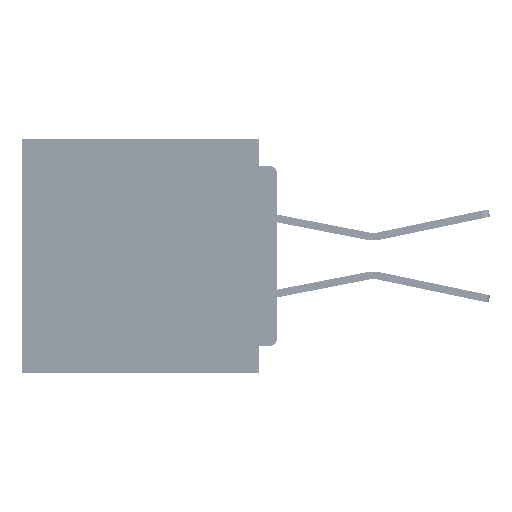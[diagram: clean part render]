
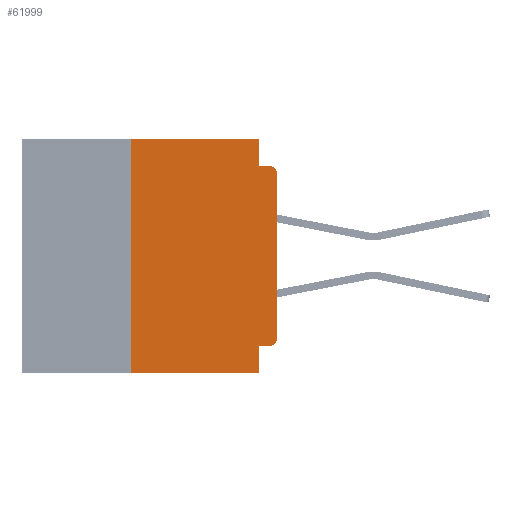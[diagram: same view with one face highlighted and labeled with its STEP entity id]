
A CAD part, left-side view. The second image highlights one B-rep face of the part: STEP entity #61999.
In plain terms, the highlighted planar face has unit normal (-1, 0, 0).
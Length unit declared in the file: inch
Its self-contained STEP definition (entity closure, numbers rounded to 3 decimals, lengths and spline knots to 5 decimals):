
#136 = CARTESIAN_POINT ( 'NONE',  ( 0., 0.25, 0. ) ) ;
#702 = DIRECTION ( 'NONE',  ( 0., 0., 1. ) ) ;
#851 = DIRECTION ( 'NONE',  ( -1., 0., 0. ) ) ;
#1193 = EDGE_CURVE ( 'NONE', #56111, #19656, #16438, .T. ) ;
#1339 = ORIENTED_EDGE ( 'NONE', *, *, #23417, .T. ) ;
#1462 = VECTOR ( 'NONE', #38180, 39.37008 ) ;
#2304 = VERTEX_POINT ( 'NONE', #56206 ) ;
#3399 = VECTOR ( 'NONE', #702, 39.37008 ) ;
#4113 = VECTOR ( 'NONE', #35135, 39.37008 ) ;
#4459 = DIRECTION ( 'NONE',  ( 1., 0., 0. ) ) ;
#5247 = ORIENTED_EDGE ( 'NONE', *, *, #41955, .F. ) ;
#6307 = EDGE_CURVE ( 'NONE', #49589, #40310, #62757, .T. ) ;
#6963 = ORIENTED_EDGE ( 'NONE', *, *, #1193, .F. ) ;
#8898 = CARTESIAN_POINT ( 'NONE',  ( 0., 0., -0.045 ) ) ;
#11327 = VERTEX_POINT ( 'NONE', #18063 ) ;
#13127 = ORIENTED_EDGE ( 'NONE', *, *, #51377, .F. ) ;
#13750 = LINE ( 'NONE', #61336, #63961 ) ;
#14013 = CIRCLE ( 'NONE', #24514, 0.015 ) ;
#14481 = ORIENTED_EDGE ( 'NONE', *, *, #58728, .F. ) ;
#15562 = VERTEX_POINT ( 'NONE', #31339 ) ;
#16078 = DIRECTION ( 'NONE',  ( -1., 0., 0. ) ) ;
#16438 = LINE ( 'NONE', #43015, #1462 ) ;
#18063 = CARTESIAN_POINT ( 'NONE',  ( 0., 0., -0.06 ) ) ;
#18684 = CARTESIAN_POINT ( 'NONE',  ( 0., 0.015, -0.045 ) ) ;
#18999 = ORIENTED_EDGE ( 'NONE', *, *, #6307, .T. ) ;
#19447 = LINE ( 'NONE', #32800, #29678 ) ;
#19462 = CARTESIAN_POINT ( 'NONE',  ( 0., 0.437, 0. ) ) ;
#19552 = CARTESIAN_POINT ( 'NONE',  ( 0., 0.031, 0. ) ) ;
#19656 = VERTEX_POINT ( 'NONE', #22319 ) ;
#21448 = FACE_OUTER_BOUND ( 'NONE', #26202, .T. ) ;
#21689 = CARTESIAN_POINT ( 'NONE',  ( 0., 0.25, -0.4 ) ) ;
#22319 = CARTESIAN_POINT ( 'NONE',  ( 0., 0.031, 0. ) ) ;
#22902 = DIRECTION ( 'NONE',  ( 0., 1., 0. ) ) ;
#23199 = CIRCLE ( 'NONE', #56171, 0.015 ) ;
#23417 = EDGE_CURVE ( 'NONE', #33600, #2304, #14013, .T. ) ;
#24514 = AXIS2_PLACEMENT_3D ( 'NONE', #46212, #16078, #51242 ) ;
#25986 = VECTOR ( 'NONE', #44781, 39.37008 ) ;
#26111 = EDGE_CURVE ( 'NONE', #2304, #11327, #31807, .T. ) ;
#26202 = EDGE_LOOP ( 'NONE', ( #62507, #61592, #13127, #57307, #6963, #5247, #18999, #32442, #14481, #1339 ) ) ;
#27563 = LINE ( 'NONE', #19552, #25986 ) ;
#29678 = VECTOR ( 'NONE', #22902, 39.37008 ) ;
#30860 = CARTESIAN_POINT ( 'NONE',  ( 0., 0.031, -0.4 ) ) ;
#31057 = CARTESIAN_POINT ( 'NONE',  ( 0., 0.015, -0.06 ) ) ;
#31339 = CARTESIAN_POINT ( 'NONE',  ( 0., 0.031, -0.355 ) ) ;
#31807 = LINE ( 'NONE', #50859, #3399 ) ;
#32442 = ORIENTED_EDGE ( 'NONE', *, *, #59871, .F. ) ;
#32800 = CARTESIAN_POINT ( 'NONE',  ( 0., 0., -0.355 ) ) ;
#33600 = VERTEX_POINT ( 'NONE', #63336 ) ;
#34626 = PLANE ( 'NONE',  #52569 ) ;
#34887 = DIRECTION ( 'NONE',  ( 0., -1., 0. ) ) ;
#35135 = DIRECTION ( 'NONE',  ( 0., 0., 1. ) ) ;
#36077 = DIRECTION ( 'NONE',  ( 0., 0., -1. ) ) ;
#36123 = VECTOR ( 'NONE', #34887, 39.37008 ) ;
#38180 = DIRECTION ( 'NONE',  ( 0., -1., 0. ) ) ;
#39653 = DIRECTION ( 'NONE',  ( 0., 0., -1. ) ) ;
#39913 = CARTESIAN_POINT ( 'NONE',  ( 0., 0.437, -0.4 ) ) ;
#40310 = VERTEX_POINT ( 'NONE', #30860 ) ;
#41955 = EDGE_CURVE ( 'NONE', #49589, #56111, #42657, .T. ) ;
#42657 = LINE ( 'NONE', #65091, #4113 ) ;
#43015 = CARTESIAN_POINT ( 'NONE',  ( 0., 0.437, 0. ) ) ;
#44037 = CARTESIAN_POINT ( 'NONE',  ( 0., 0.031, -0.045 ) ) ;
#44781 = DIRECTION ( 'NONE',  ( 0., 0., -1. ) ) ;
#46212 = CARTESIAN_POINT ( 'NONE',  ( 0., 0.015, -0.34 ) ) ;
#48333 = EDGE_CURVE ( 'NONE', #11327, #53420, #23199, .T. ) ;
#49589 = VERTEX_POINT ( 'NONE', #21689 ) ;
#50845 = VECTOR ( 'NONE', #59130, 39.37008 ) ;
#50859 = CARTESIAN_POINT ( 'NONE',  ( 0., 0., 0. ) ) ;
#51242 = DIRECTION ( 'NONE',  ( 0., 0., -1. ) ) ;
#51377 = EDGE_CURVE ( 'NONE', #57224, #53420, #64106, .T. ) ;
#51539 = DIRECTION ( 'NONE',  ( 0., 0., -1. ) ) ;
#52569 = AXIS2_PLACEMENT_3D ( 'NONE', #19462, #4459, #39653 ) ;
#53420 = VERTEX_POINT ( 'NONE', #18684 ) ;
#56111 = VERTEX_POINT ( 'NONE', #136 ) ;
#56171 = AXIS2_PLACEMENT_3D ( 'NONE', #31057, #851, #36077 ) ;
#56206 = CARTESIAN_POINT ( 'NONE',  ( 0., 0., -0.34 ) ) ;
#57224 = VERTEX_POINT ( 'NONE', #44037 ) ;
#57307 = ORIENTED_EDGE ( 'NONE', *, *, #63230, .F. ) ;
#58728 = EDGE_CURVE ( 'NONE', #33600, #15562, #19447, .T. ) ;
#59130 = DIRECTION ( 'NONE',  ( 0., -1., 0. ) ) ;
#59871 = EDGE_CURVE ( 'NONE', #15562, #40310, #13750, .T. ) ;
#61336 = CARTESIAN_POINT ( 'NONE',  ( 0., 0.031, -0.4 ) ) ;
#61592 = ORIENTED_EDGE ( 'NONE', *, *, #48333, .T. ) ;
#61999 = ADVANCED_FACE ( 'NONE', ( #21448 ), #34626, .F. ) ;
#62507 = ORIENTED_EDGE ( 'NONE', *, *, #26111, .T. ) ;
#62757 = LINE ( 'NONE', #39913, #36123 ) ;
#63230 = EDGE_CURVE ( 'NONE', #19656, #57224, #27563, .T. ) ;
#63336 = CARTESIAN_POINT ( 'NONE',  ( 0., 0.015, -0.355 ) ) ;
#63961 = VECTOR ( 'NONE', #51539, 39.37008 ) ;
#64106 = LINE ( 'NONE', #8898, #50845 ) ;
#65091 = CARTESIAN_POINT ( 'NONE',  ( 0., 0.25, -0.4 ) ) ;
